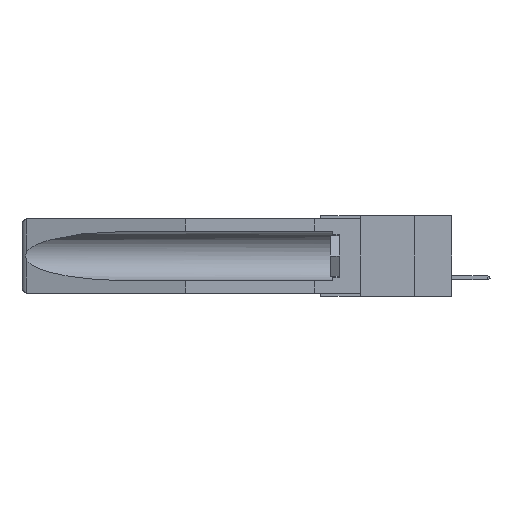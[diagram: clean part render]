
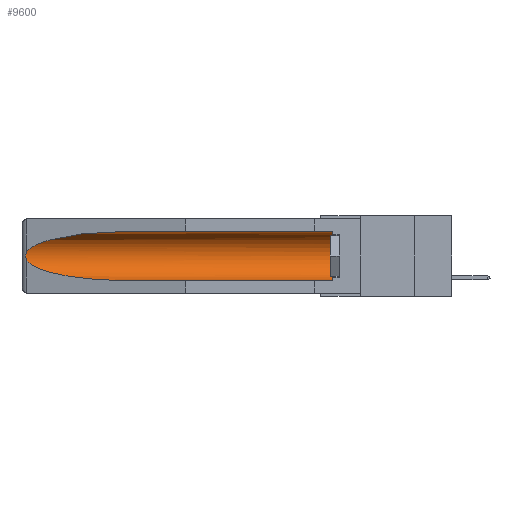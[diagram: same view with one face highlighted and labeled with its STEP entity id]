
A CAD part, left-side view. The second image highlights one B-rep face of the part: STEP entity #9600.
In plain terms, the highlighted cylindrical face has radius 2.857 mm (diameter 5.715 mm), a partial arc.
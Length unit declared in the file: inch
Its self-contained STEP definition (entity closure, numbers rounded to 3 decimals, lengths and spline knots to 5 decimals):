
#121 = AXIS2_PLACEMENT_3D ( 'NONE', #28940, #8536, #31358 ) ;
#137 = DIRECTION ( 'NONE',  ( 0., 1., 0. ) ) ;
#480 = DIRECTION ( 'NONE',  ( 0., 0., 1. ) ) ;
#2161 = EDGE_CURVE ( 'NONE', #15489, #7816, #31872, .T. ) ;
#2541 = CARTESIAN_POINT ( 'NONE',  ( 0.25451, 1.48313, -0.24835 ) ) ;
#2596 = ORIENTED_EDGE ( 'NONE', *, *, #14324, .T. ) ;
#3050 = VECTOR ( 'NONE', #137, 39.37008 ) ;
#3055 = ORIENTED_EDGE ( 'NONE', *, *, #14654, .F. ) ;
#4058 = CARTESIAN_POINT ( 'NONE',  ( 0.26537, 1.52718, -0.14972 ) ) ;
#4163 = CARTESIAN_POINT ( 'NONE',  ( 0.26597, 1.5296, -0.19026 ) ) ;
#4751 =( BOUNDED_CURVE ( )  B_SPLINE_CURVE ( 3, ( #9610, #2541, #27695, #20170 ),
 .UNSPECIFIED., .F., .F. ) 
 B_SPLINE_CURVE_WITH_KNOTS ( ( 4, 4 ),
 ( 0.1948, 1.5708 ),
 .UNSPECIFIED. ) 
 CURVE ( )  GEOMETRIC_REPRESENTATION_ITEM ( )  RATIONAL_B_SPLINE_CURVE ( ( 1., 0.848, 0.848, 1. ) ) 
 REPRESENTATION_ITEM ( '' )  );
#6249 = VERTEX_POINT ( 'NONE', #32548 ) ;
#7190 = FACE_OUTER_BOUND ( 'NONE', #22765, .T. ) ;
#7806 = CARTESIAN_POINT ( 'NONE',  ( 0.155, -0.30754, -0.059 ) ) ;
#7816 = VERTEX_POINT ( 'NONE', #22074 ) ;
#8536 = DIRECTION ( 'NONE',  ( 0., 1., 0. ) ) ;
#8583 = CARTESIAN_POINT ( 'NONE',  ( 0.26537, 1.52718, -0.14972 ) ) ;
#9110 = CARTESIAN_POINT ( 'NONE',  ( 0.26655, 1.53094, -0.18657 ) ) ;
#9600 = ADVANCED_FACE ( 'NONE', ( #7190 ), #22577, .F. ) ;
#9610 = CARTESIAN_POINT ( 'NONE',  ( 0.26537, 1.52718, -0.19328 ) ) ;
#9619 =( BOUNDED_CURVE ( )  B_SPLINE_CURVE ( 3, ( #29428, #16520, #29215, #11769 ),
 .UNSPECIFIED., .F., .F. ) 
 B_SPLINE_CURVE_WITH_KNOTS ( ( 4, 4 ),
 ( 4.71239, 6.08839 ),
 .UNSPECIFIED. ) 
 CURVE ( )  GEOMETRIC_REPRESENTATION_ITEM ( )  RATIONAL_B_SPLINE_CURVE ( ( 1., 0.848, 0.848, 1. ) ) 
 REPRESENTATION_ITEM ( '' )  );
#11395 = CIRCLE ( 'NONE', #28652, 0.1125 ) ;
#11769 = CARTESIAN_POINT ( 'NONE',  ( 0.26537, 1.52718, -0.14972 ) ) ;
#12221 = DIRECTION ( 'NONE',  ( 0., 1., 0. ) ) ;
#12940 = VECTOR ( 'NONE', #12221, 39.37008 ) ;
#13312 = VERTEX_POINT ( 'NONE', #8583 ) ;
#14324 = EDGE_CURVE ( 'NONE', #26404, #15489, #11395, .T. ) ;
#14654 = EDGE_CURVE ( 'NONE', #26404, #6249, #18475, .T. ) ;
#15489 = VERTEX_POINT ( 'NONE', #28377 ) ;
#16505 = CARTESIAN_POINT ( 'NONE',  ( 0.2675, 1.53308, -0.16763 ) ) ;
#16520 = CARTESIAN_POINT ( 'NONE',  ( 0.21114, 1.30732, -0.059 ) ) ;
#17462 = EDGE_CURVE ( 'NONE', #7816, #13312, #9619, .T. ) ;
#18105 = CARTESIAN_POINT ( 'NONE',  ( 0.155, 0.126, -0.284 ) ) ;
#18475 = LINE ( 'NONE', #29980, #12940 ) ;
#19045 = CARTESIAN_POINT ( 'NONE',  ( 0.2675, 1.53308, -0.17534 ) ) ;
#19259 = CARTESIAN_POINT ( 'NONE',  ( 0.2673, 1.5327, -0.16383 ) ) ;
#20170 = CARTESIAN_POINT ( 'NONE',  ( 0.155, 1.07973, -0.284 ) ) ;
#21450 = ORIENTED_EDGE ( 'NONE', *, *, #30110, .T. ) ;
#21581 = CARTESIAN_POINT ( 'NONE',  ( 0.26654, 1.53092, -0.15636 ) ) ;
#21691 = CARTESIAN_POINT ( 'NONE',  ( 0.2673, 1.53269, -0.17917 ) ) ;
#21893 = VERTEX_POINT ( 'NONE', #27941 ) ;
#22074 = CARTESIAN_POINT ( 'NONE',  ( 0.155, 1.07973, -0.059 ) ) ;
#22372 = B_SPLINE_CURVE_WITH_KNOTS ( 'NONE', 3,
 ( #4058, #29086, #21581, #19259, #16505, #19045, #21691, #9110, #4163, #29411 ),
 .UNSPECIFIED., .F., .F.,
 ( 4, 2, 2, 2, 4 ),
 ( 0., 0.00029, 0.00058, 0.00087, 0.00117 ),
 .UNSPECIFIED. ) ;
#22577 = CYLINDRICAL_SURFACE ( 'NONE', #121, 0.1125 ) ;
#22765 = EDGE_LOOP ( 'NONE', ( #25579, #24754, #21450, #3055, #2596, #27659 ) ) ;
#22915 = EDGE_CURVE ( 'NONE', #13312, #21893, #22372, .T. ) ;
#24754 = ORIENTED_EDGE ( 'NONE', *, *, #22915, .T. ) ;
#25579 = ORIENTED_EDGE ( 'NONE', *, *, #17462, .T. ) ;
#25824 = DIRECTION ( 'NONE',  ( 0., -1., 0. ) ) ;
#26404 = VERTEX_POINT ( 'NONE', #18105 ) ;
#27659 = ORIENTED_EDGE ( 'NONE', *, *, #2161, .T. ) ;
#27695 = CARTESIAN_POINT ( 'NONE',  ( 0.21114, 1.30732, -0.284 ) ) ;
#27941 = CARTESIAN_POINT ( 'NONE',  ( 0.26537, 1.52718, -0.19328 ) ) ;
#28377 = CARTESIAN_POINT ( 'NONE',  ( 0.155, 0.126, -0.059 ) ) ;
#28652 = AXIS2_PLACEMENT_3D ( 'NONE', #30666, #25824, #480 ) ;
#28940 = CARTESIAN_POINT ( 'NONE',  ( 0.155, -0.30754, -0.1715 ) ) ;
#29086 = CARTESIAN_POINT ( 'NONE',  ( 0.26597, 1.52961, -0.15275 ) ) ;
#29215 = CARTESIAN_POINT ( 'NONE',  ( 0.25451, 1.48313, -0.09465 ) ) ;
#29411 = CARTESIAN_POINT ( 'NONE',  ( 0.26537, 1.52718, -0.19328 ) ) ;
#29428 = CARTESIAN_POINT ( 'NONE',  ( 0.155, 1.07973, -0.059 ) ) ;
#29980 = CARTESIAN_POINT ( 'NONE',  ( 0.155, -0.30754, -0.284 ) ) ;
#30110 = EDGE_CURVE ( 'NONE', #21893, #6249, #4751, .T. ) ;
#30666 = CARTESIAN_POINT ( 'NONE',  ( 0.155, 0.126, -0.1715 ) ) ;
#31358 = DIRECTION ( 'NONE',  ( 0., 0., 1. ) ) ;
#31872 = LINE ( 'NONE', #7806, #3050 ) ;
#32548 = CARTESIAN_POINT ( 'NONE',  ( 0.155, 1.07973, -0.284 ) ) ;
